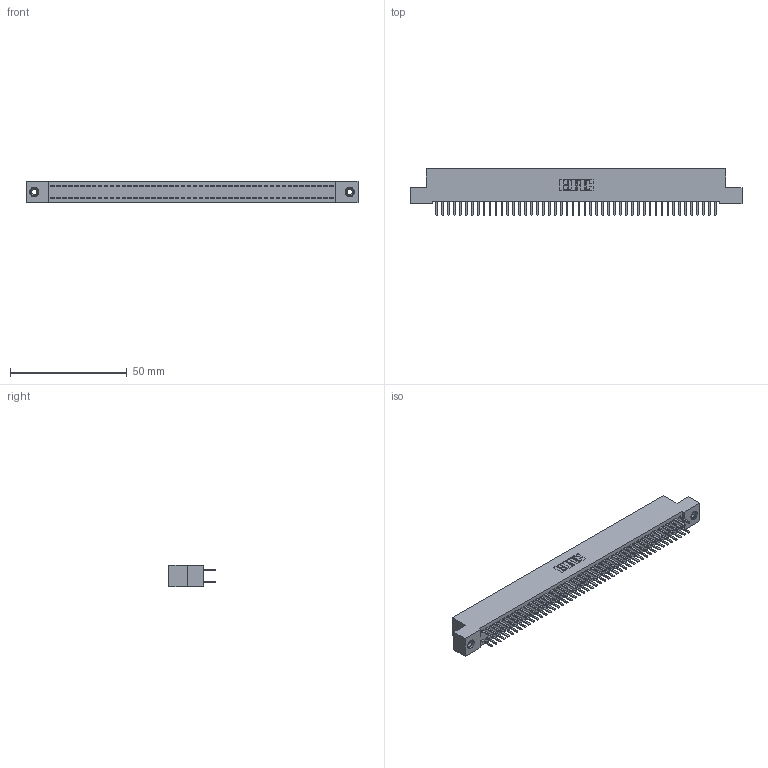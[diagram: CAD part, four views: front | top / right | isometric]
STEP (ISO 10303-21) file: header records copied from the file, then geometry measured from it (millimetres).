
FILE_DESCRIPTION (( 'STEP AP203' ), '1' );
FILE_NAME ('392-096-520-208.STEP', '2018-08-18T09:33:25', ( '' ), ( '' ), 'SwSTEP 2.0', 'SolidWorks 2016', '' );
FILE_SCHEMA (( 'CONFIG_CONTROL_DESIGN' ));
Length unit declared in the file: inch
Products named in the file (4): 342 Part_TI; 345-292-001_345-293-120; 345-250-001_345-250-003-102; 392-096-520-208
Assembly tree (99 placements, depth 2):
  392-096-520-208
    342 Part_TI
    345-292-001_345-293-120  x96
    345-250-001_345-250-003-102  x2
Bounding box: 142.24 x 20.02 x 9.4 mm (x, y, z)
Volume: 12760.8 mm3; surface area: 20829.9 mm2
Topology: 99 solids, 99 shells, 5546 faces, 16083 edges, 10458 vertices
Faces by surface type: plane 3746, cylinder 1784, cone 12, torus 4
Entity records: 31272 total; most frequent: CARTESIAN_POINT 5169, ORIENTED_EDGE 5086, DIRECTION 4425, EDGE_CURVE 2543, VECTOR 2391, LINE 2391, VERTEX_POINT 1688, AXIS2_PLACEMENT_3D 1017
